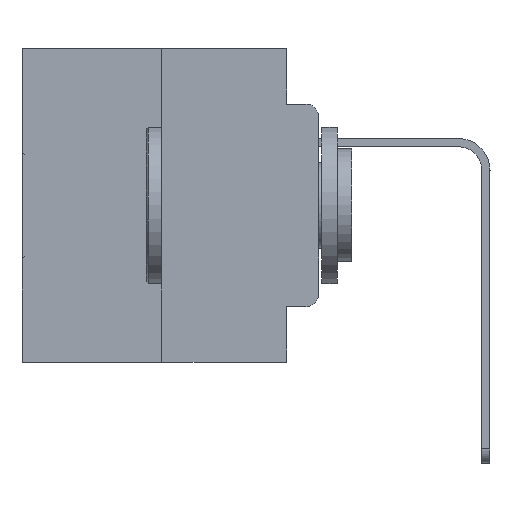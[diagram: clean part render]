
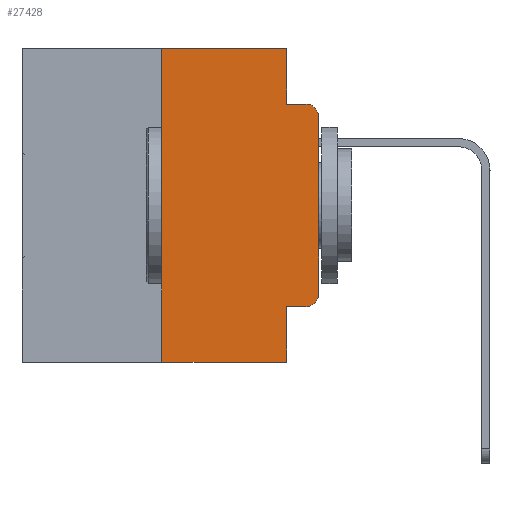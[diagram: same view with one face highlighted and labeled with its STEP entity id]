
A CAD part, left-side view. The second image highlights one B-rep face of the part: STEP entity #27428.
In plain terms, the highlighted planar face has unit normal (-1, 0, 0).
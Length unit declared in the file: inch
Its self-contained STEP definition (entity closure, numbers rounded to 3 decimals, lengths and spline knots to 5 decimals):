
#960 = VECTOR ( 'NONE', #24173, 39.37008 ) ;
#1133 = CARTESIAN_POINT ( 'NONE',  ( 0., 0.25, 0. ) ) ;
#1306 = LINE ( 'NONE', #20243, #18984 ) ;
#1625 = DIRECTION ( 'NONE',  ( -1., 0., 0. ) ) ;
#2094 = VERTEX_POINT ( 'NONE', #13907 ) ;
#2124 = ORIENTED_EDGE ( 'NONE', *, *, #22984, .T. ) ;
#2935 = LINE ( 'NONE', #25232, #4711 ) ;
#3212 = DIRECTION ( 'NONE',  ( 0., 0., -1. ) ) ;
#3390 = VERTEX_POINT ( 'NONE', #13972 ) ;
#3444 = EDGE_LOOP ( 'NONE', ( #27668, #2124, #22167, #5650, #6158, #19479, #18803, #4873, #9099, #8040 ) ) ;
#3843 = CARTESIAN_POINT ( 'NONE',  ( 0., 0.051, -0.4115 ) ) ;
#3988 = FACE_OUTER_BOUND ( 'NONE', #3444, .T. ) ;
#4443 = LINE ( 'NONE', #6825, #17062 ) ;
#4711 = VECTOR ( 'NONE', #4833, 39.37008 ) ;
#4833 = DIRECTION ( 'NONE',  ( 0., 0., 1. ) ) ;
#4873 = ORIENTED_EDGE ( 'NONE', *, *, #15092, .F. ) ;
#4990 = LINE ( 'NONE', #13698, #15132 ) ;
#5205 = EDGE_CURVE ( 'NONE', #18051, #24865, #2935, .T. ) ;
#5247 = CARTESIAN_POINT ( 'NONE',  ( 0., 0.051, 0. ) ) ;
#5435 = EDGE_CURVE ( 'NONE', #2094, #12768, #7588, .T. ) ;
#5650 = ORIENTED_EDGE ( 'NONE', *, *, #25351, .F. ) ;
#5841 = CARTESIAN_POINT ( 'NONE',  ( 0., 0.25, 0. ) ) ;
#6158 = ORIENTED_EDGE ( 'NONE', *, *, #9205, .F. ) ;
#6213 = EDGE_CURVE ( 'NONE', #2094, #16263, #4990, .T. ) ;
#6609 = VERTEX_POINT ( 'NONE', #15908 ) ;
#6825 = CARTESIAN_POINT ( 'NONE',  ( 0., 0.051, 0. ) ) ;
#7588 = LINE ( 'NONE', #5841, #21638 ) ;
#8040 = ORIENTED_EDGE ( 'NONE', *, *, #14600, .T. ) ;
#8618 = CARTESIAN_POINT ( 'NONE',  ( 0., 0.02, -0.3915 ) ) ;
#9099 = ORIENTED_EDGE ( 'NONE', *, *, #29002, .T. ) ;
#9205 = EDGE_CURVE ( 'NONE', #12768, #28759, #13250, .T. ) ;
#9529 = EDGE_CURVE ( 'NONE', #3390, #6609, #1306, .T. ) ;
#9977 = CARTESIAN_POINT ( 'NONE',  ( 0., 0.473, 0. ) ) ;
#11509 = VECTOR ( 'NONE', #19991, 39.37008 ) ;
#12395 = CARTESIAN_POINT ( 'NONE',  ( 0., 0.473, 0. ) ) ;
#12768 = VERTEX_POINT ( 'NONE', #1133 ) ;
#13250 = LINE ( 'NONE', #9977, #960 ) ;
#13515 = DIRECTION ( 'NONE',  ( 0., -1., 0. ) ) ;
#13607 = LINE ( 'NONE', #19752, #26548 ) ;
#13698 = CARTESIAN_POINT ( 'NONE',  ( 0., 0.473, -0.5 ) ) ;
#13902 = DIRECTION ( 'NONE',  ( 0., 0., -1. ) ) ;
#13907 = CARTESIAN_POINT ( 'NONE',  ( 0., 0.25, -0.5 ) ) ;
#13972 = CARTESIAN_POINT ( 'NONE',  ( 0., 0.051, -0.0885 ) ) ;
#14019 = CARTESIAN_POINT ( 'NONE',  ( 0., 0.051, -0.5 ) ) ;
#14413 = CARTESIAN_POINT ( 'NONE',  ( 0., 0., -0.3915 ) ) ;
#14600 = EDGE_CURVE ( 'NONE', #29805, #18051, #27296, .T. ) ;
#15031 = DIRECTION ( 'NONE',  ( 0., 0., -1. ) ) ;
#15092 = EDGE_CURVE ( 'NONE', #17842, #16263, #13607, .T. ) ;
#15132 = VECTOR ( 'NONE', #22934, 39.37008 ) ;
#15540 = CARTESIAN_POINT ( 'NONE',  ( 0., 0.051, -0.4115 ) ) ;
#15908 = CARTESIAN_POINT ( 'NONE',  ( 0., 0.02, -0.0885 ) ) ;
#16263 = VERTEX_POINT ( 'NONE', #14019 ) ;
#17025 = DIRECTION ( 'NONE',  ( 1., 0., 0. ) ) ;
#17062 = VECTOR ( 'NONE', #13902, 39.37008 ) ;
#17842 = VERTEX_POINT ( 'NONE', #15540 ) ;
#18051 = VERTEX_POINT ( 'NONE', #14413 ) ;
#18179 = CARTESIAN_POINT ( 'NONE',  ( 0., 0.02, -0.1085 ) ) ;
#18803 = ORIENTED_EDGE ( 'NONE', *, *, #6213, .T. ) ;
#18984 = VECTOR ( 'NONE', #13515, 39.37008 ) ;
#19479 = ORIENTED_EDGE ( 'NONE', *, *, #5435, .F. ) ;
#19752 = CARTESIAN_POINT ( 'NONE',  ( 0., 0.051, 0. ) ) ;
#19954 = CARTESIAN_POINT ( 'NONE',  ( 0., 0., -0.1085 ) ) ;
#19991 = DIRECTION ( 'NONE',  ( 0., -1., 0. ) ) ;
#20188 = DIRECTION ( 'NONE',  ( 0., 0., -1. ) ) ;
#20243 = CARTESIAN_POINT ( 'NONE',  ( 0., 0.051, -0.0885 ) ) ;
#20831 = AXIS2_PLACEMENT_3D ( 'NONE', #18179, #21167, #25514 ) ;
#21167 = DIRECTION ( 'NONE',  ( -1., 0., 0. ) ) ;
#21638 = VECTOR ( 'NONE', #29083, 39.37008 ) ;
#22167 = ORIENTED_EDGE ( 'NONE', *, *, #9529, .F. ) ;
#22674 = LINE ( 'NONE', #3843, #11509 ) ;
#22934 = DIRECTION ( 'NONE',  ( 0., -1., 0. ) ) ;
#22984 = EDGE_CURVE ( 'NONE', #24865, #6609, #24064, .T. ) ;
#24064 = CIRCLE ( 'NONE', #20831, 0.02 ) ;
#24169 = AXIS2_PLACEMENT_3D ( 'NONE', #12395, #17025, #3212 ) ;
#24173 = DIRECTION ( 'NONE',  ( 0., -1., 0. ) ) ;
#24865 = VERTEX_POINT ( 'NONE', #19954 ) ;
#24967 = AXIS2_PLACEMENT_3D ( 'NONE', #8618, #1625, #20188 ) ;
#25232 = CARTESIAN_POINT ( 'NONE',  ( 0., 0., 0. ) ) ;
#25351 = EDGE_CURVE ( 'NONE', #28759, #3390, #4443, .T. ) ;
#25514 = DIRECTION ( 'NONE',  ( 0., 0., -1. ) ) ;
#26548 = VECTOR ( 'NONE', #15031, 39.37008 ) ;
#26563 = PLANE ( 'NONE',  #24169 ) ;
#27296 = CIRCLE ( 'NONE', #24967, 0.02 ) ;
#27428 = ADVANCED_FACE ( 'NONE', ( #3988 ), #26563, .F. ) ;
#27668 = ORIENTED_EDGE ( 'NONE', *, *, #5205, .T. ) ;
#28759 = VERTEX_POINT ( 'NONE', #5247 ) ;
#29002 = EDGE_CURVE ( 'NONE', #17842, #29805, #22674, .T. ) ;
#29083 = DIRECTION ( 'NONE',  ( 0., 0., 1. ) ) ;
#29317 = CARTESIAN_POINT ( 'NONE',  ( 0., 0.02, -0.4115 ) ) ;
#29805 = VERTEX_POINT ( 'NONE', #29317 ) ;
